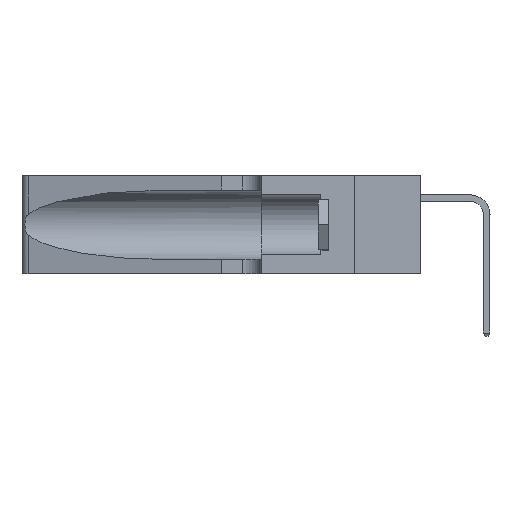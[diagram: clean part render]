
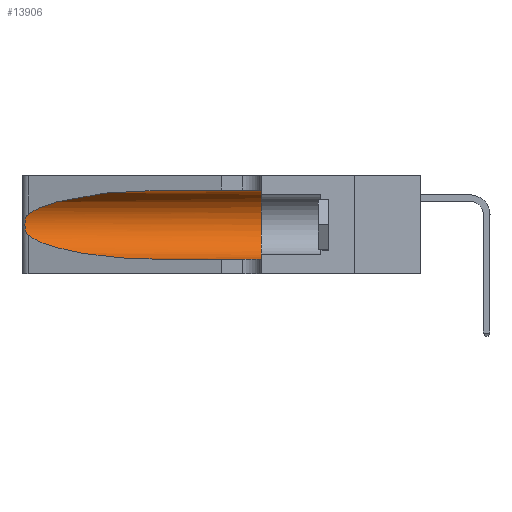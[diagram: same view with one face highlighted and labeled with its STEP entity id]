
A CAD part, left-side view. The second image highlights one B-rep face of the part: STEP entity #13906.
In plain terms, the highlighted cylindrical face has radius 3.308 mm (diameter 6.617 mm), a partial arc.
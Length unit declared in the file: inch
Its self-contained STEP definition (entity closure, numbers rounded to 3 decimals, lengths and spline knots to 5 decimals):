
#605 = CARTESIAN_POINT ( 'NONE',  ( 0.25487, 1.22718, 0.14631 ) ) ;
#1382 = CARTESIAN_POINT ( 'NONE',  ( 0.26017, 1.23833, 0.17102 ) ) ;
#2775 = VECTOR ( 'NONE', #17752, 39.37008 ) ;
#3429 = CARTESIAN_POINT ( 'NONE',  ( 0.25789, 1.23486, 0.15765 ) ) ;
#3508 = AXIS2_PLACEMENT_3D ( 'NONE', #13136, #19092, #7232 ) ;
#3658 = EDGE_CURVE ( 'NONE', #19532, #19113, #23271, .T. ) ;
#4039 = CARTESIAN_POINT ( 'NONE',  ( 0.1305, 0.72297, 0.31525 ) ) ;
#4358 = ORIENTED_EDGE ( 'NONE', *, *, #3658, .T. ) ;
#5233 = AXIS2_PLACEMENT_3D ( 'NONE', #8567, #22364, #10576 ) ;
#5390 = CARTESIAN_POINT ( 'NONE',  ( 0.25487, 1.22718, 0.22369 ) ) ;
#5478 = CARTESIAN_POINT ( 'NONE',  ( 0.25555, 1.22993, 0.14849 ) ) ;
#5722 = CARTESIAN_POINT ( 'NONE',  ( 0.1305, 0.72297, 0.05475 ) ) ;
#5934 = CARTESIAN_POINT ( 'NONE',  ( 0.1305, 1.61858, 0.05475 ) ) ;
#5968 = LINE ( 'NONE', #11618, #10065 ) ;
#6899 = B_SPLINE_CURVE_WITH_KNOTS ( 'NONE', 3,
 ( #5390, #17282, #21225, #9423, #23216, #11414, #25221, #13371, #1382, #15371, #3429, #17361, #5478, #19326 ),
 .UNSPECIFIED., .F., .F.,
 ( 4, 2, 2, 2, 2, 2, 4 ),
 ( 0., 0.00027, 0.00053, 0.00107, 0.0016, 0.00187, 0.00214 ),
 .UNSPECIFIED. ) ;
#6973 = VERTEX_POINT ( 'NONE', #22516 ) ;
#7172 = ORIENTED_EDGE ( 'NONE', *, *, #18830, .F. ) ;
#7232 = DIRECTION ( 'NONE',  ( 0., 0., -1. ) ) ;
#7814 = CIRCLE ( 'NONE', #5233, 0.13025 ) ;
#8567 = CARTESIAN_POINT ( 'NONE',  ( 0.1305, 0.35, 0.185 ) ) ;
#8852 = CARTESIAN_POINT ( 'NONE',  ( 0.1305, 0.72297, 0.31525 ) ) ;
#9016 = ORIENTED_EDGE ( 'NONE', *, *, #16400, .T. ) ;
#9043 = CARTESIAN_POINT ( 'NONE',  ( 0.25487, 1.22718, 0.22369 ) ) ;
#9423 = CARTESIAN_POINT ( 'NONE',  ( 0.25787, 1.23484, 0.2124 ) ) ;
#10065 = VECTOR ( 'NONE', #23338, 39.37008 ) ;
#10500 = EDGE_CURVE ( 'NONE', #19292, #19532, #17052, .T. ) ;
#10576 = DIRECTION ( 'NONE',  ( 0., 0., 1. ) ) ;
#10656 = CARTESIAN_POINT ( 'NONE',  ( 0.18966, 0.96281, 0.05475 ) ) ;
#10704 = EDGE_CURVE ( 'NONE', #15127, #19292, #6899, .T. ) ;
#11164 =( BOUNDED_CURVE ( )  B_SPLINE_CURVE ( 3, ( #8852, #20659, #24642, #12813 ),
 .UNSPECIFIED., .F., .T. ) 
 B_SPLINE_CURVE_WITH_KNOTS ( ( 4, 4 ),
 ( 1.5708, 2.84003 ),
 .UNSPECIFIED. ) 
 CURVE ( )  GEOMETRIC_REPRESENTATION_ITEM ( )  RATIONAL_B_SPLINE_CURVE ( ( 1., 0.87, 0.87, 1. ) ) 
 REPRESENTATION_ITEM ( '' )  );
#11414 = CARTESIAN_POINT ( 'NONE',  ( 0.26018, 1.23835, 0.19895 ) ) ;
#11448 = VERTEX_POINT ( 'NONE', #4039 ) ;
#11618 = CARTESIAN_POINT ( 'NONE',  ( 0.1305, 1.61858, 0.31525 ) ) ;
#12614 = CARTESIAN_POINT ( 'NONE',  ( 0.2373, 1.15595, 0.08982 ) ) ;
#12813 = CARTESIAN_POINT ( 'NONE',  ( 0.25487, 1.22718, 0.22369 ) ) ;
#13136 = CARTESIAN_POINT ( 'NONE',  ( 0.1305, 1.61858, 0.185 ) ) ;
#13371 = CARTESIAN_POINT ( 'NONE',  ( 0.26075, 1.23896, 0.178 ) ) ;
#13906 = ADVANCED_FACE ( 'NONE', ( #25131 ), #18620, .F. ) ;
#14455 = ORIENTED_EDGE ( 'NONE', *, *, #10704, .T. ) ;
#14578 = CARTESIAN_POINT ( 'NONE',  ( 0.1305, 0.72297, 0.05475 ) ) ;
#15127 = VERTEX_POINT ( 'NONE', #9043 ) ;
#15371 = CARTESIAN_POINT ( 'NONE',  ( 0.25856, 1.23593, 0.16098 ) ) ;
#15534 = ORIENTED_EDGE ( 'NONE', *, *, #25158, .F. ) ;
#16400 = EDGE_CURVE ( 'NONE', #11448, #15127, #11164, .T. ) ;
#16442 = CARTESIAN_POINT ( 'NONE',  ( 0.1305, 0.35, 0.05475 ) ) ;
#17052 =( BOUNDED_CURVE ( )  B_SPLINE_CURVE ( 3, ( #605, #12614, #10656, #14578 ),
 .UNSPECIFIED., .F., .F. ) 
 B_SPLINE_CURVE_WITH_KNOTS ( ( 4, 4 ),
 ( 3.44316, 4.71239 ),
 .UNSPECIFIED. ) 
 CURVE ( )  GEOMETRIC_REPRESENTATION_ITEM ( )  RATIONAL_B_SPLINE_CURVE ( ( 1., 0.87, 0.87, 1. ) ) 
 REPRESENTATION_ITEM ( '' )  );
#17282 = CARTESIAN_POINT ( 'NONE',  ( 0.25555, 1.22994, 0.2215 ) ) ;
#17361 = CARTESIAN_POINT ( 'NONE',  ( 0.25639, 1.23186, 0.15144 ) ) ;
#17752 = DIRECTION ( 'NONE',  ( 0., -1., 0. ) ) ;
#18620 = CYLINDRICAL_SURFACE ( 'NONE', #3508, 0.13025 ) ;
#18830 = EDGE_CURVE ( 'NONE', #11448, #6973, #5968, .T. ) ;
#18896 = CARTESIAN_POINT ( 'NONE',  ( 0.25487, 1.22718, 0.14631 ) ) ;
#19092 = DIRECTION ( 'NONE',  ( 0., -1., 0. ) ) ;
#19113 = VERTEX_POINT ( 'NONE', #16442 ) ;
#19292 = VERTEX_POINT ( 'NONE', #18896 ) ;
#19326 = CARTESIAN_POINT ( 'NONE',  ( 0.25487, 1.22718, 0.14631 ) ) ;
#19532 = VERTEX_POINT ( 'NONE', #5722 ) ;
#20659 = CARTESIAN_POINT ( 'NONE',  ( 0.18966, 0.96281, 0.31525 ) ) ;
#21083 = EDGE_LOOP ( 'NONE', ( #9016, #14455, #21280, #4358, #15534, #7172 ) ) ;
#21225 = CARTESIAN_POINT ( 'NONE',  ( 0.25639, 1.23184, 0.21858 ) ) ;
#21280 = ORIENTED_EDGE ( 'NONE', *, *, #10500, .T. ) ;
#22364 = DIRECTION ( 'NONE',  ( 0., 1., 0. ) ) ;
#22516 = CARTESIAN_POINT ( 'NONE',  ( 0.1305, 0.35, 0.31525 ) ) ;
#23216 = CARTESIAN_POINT ( 'NONE',  ( 0.25854, 1.2359, 0.20912 ) ) ;
#23271 = LINE ( 'NONE', #5934, #2775 ) ;
#23338 = DIRECTION ( 'NONE',  ( 0., -1., 0. ) ) ;
#24642 = CARTESIAN_POINT ( 'NONE',  ( 0.2373, 1.15595, 0.28018 ) ) ;
#25131 = FACE_OUTER_BOUND ( 'NONE', #21083, .T. ) ;
#25158 = EDGE_CURVE ( 'NONE', #6973, #19113, #7814, .T. ) ;
#25221 = CARTESIAN_POINT ( 'NONE',  ( 0.26075, 1.23896, 0.19203 ) ) ;
